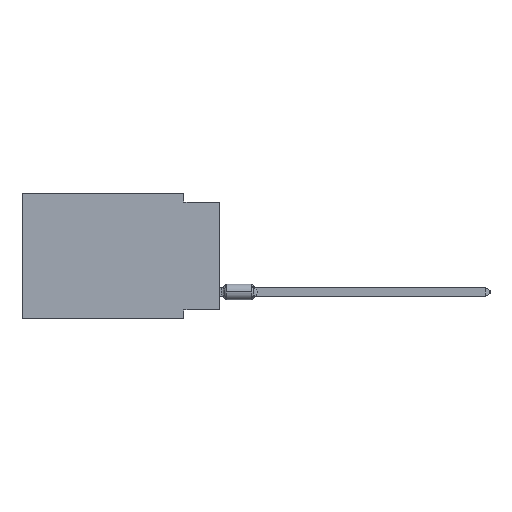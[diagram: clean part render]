
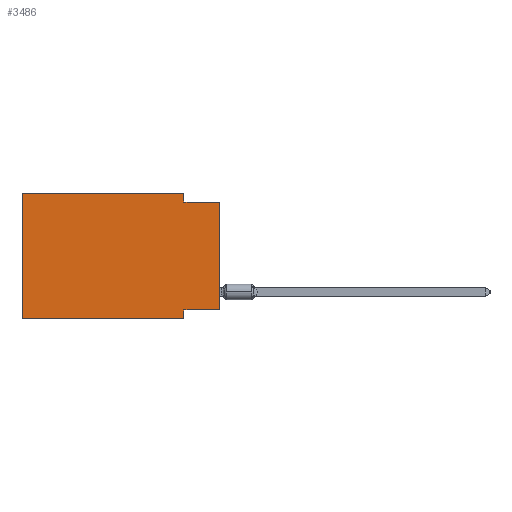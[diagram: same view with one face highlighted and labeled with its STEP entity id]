
A CAD part, left-side view. The second image highlights one B-rep face of the part: STEP entity #3486.
In plain terms, the highlighted planar face has unit normal (-1, 0, 0).
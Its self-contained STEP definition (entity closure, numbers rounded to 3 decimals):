
#558 = EDGE_CURVE ( 'NONE', #11750, #9548, #14849, .T. ) ;
#1206 = PLANE ( 'NONE',  #18500 ) ;
#1354 = DIRECTION ( 'NONE',  ( 0., -1., 0. ) ) ;
#1635 = VECTOR ( 'NONE', #8632, 1000. ) ;
#1766 = CARTESIAN_POINT ( 'NONE',  ( 0., 13.97, 0. ) ) ;
#2144 = CARTESIAN_POINT ( 'NONE',  ( 0., 2.54, -8.89 ) ) ;
#2290 = VECTOR ( 'NONE', #11818, 1000. ) ;
#2728 = CARTESIAN_POINT ( 'NONE',  ( 0., 2.54, -8.89 ) ) ;
#3170 = ORIENTED_EDGE ( 'NONE', *, *, #18254, .F. ) ;
#3486 = ADVANCED_FACE ( 'NONE', ( #5914 ), #1206, .F. ) ;
#3530 = EDGE_CURVE ( 'NONE', #15870, #7980, #17736, .T. ) ;
#3556 = LINE ( 'NONE', #18322, #11150 ) ;
#4322 = ORIENTED_EDGE ( 'NONE', *, *, #18284, .F. ) ;
#4835 = EDGE_CURVE ( 'NONE', #9548, #13205, #13509, .T. ) ;
#5208 = LINE ( 'NONE', #8612, #12692 ) ;
#5242 = CARTESIAN_POINT ( 'NONE',  ( 0., 2.54, -8.255 ) ) ;
#5760 = CARTESIAN_POINT ( 'NONE',  ( 0., 0., -0.635 ) ) ;
#5914 = FACE_OUTER_BOUND ( 'NONE', #9506, .T. ) ;
#6008 = CARTESIAN_POINT ( 'NONE',  ( 0., 2.54, 0. ) ) ;
#6281 = VECTOR ( 'NONE', #16635, 1000. ) ;
#6941 = VERTEX_POINT ( 'NONE', #5242 ) ;
#7406 = LINE ( 'NONE', #8763, #11508 ) ;
#7618 = CARTESIAN_POINT ( 'NONE',  ( 0., 0., -0.635 ) ) ;
#7980 = VERTEX_POINT ( 'NONE', #7618 ) ;
#8101 = DIRECTION ( 'NONE',  ( 0., 0., -1. ) ) ;
#8123 = ORIENTED_EDGE ( 'NONE', *, *, #8288, .T. ) ;
#8288 = EDGE_CURVE ( 'NONE', #11750, #16385, #7406, .T. ) ;
#8612 = CARTESIAN_POINT ( 'NONE',  ( 0., 0., -8.255 ) ) ;
#8632 = DIRECTION ( 'NONE',  ( 0., 0., 1. ) ) ;
#8695 = ORIENTED_EDGE ( 'NONE', *, *, #16436, .F. ) ;
#8763 = CARTESIAN_POINT ( 'NONE',  ( 0., 13.97, -8.89 ) ) ;
#8831 = DIRECTION ( 'NONE',  ( 1., 0., 0. ) ) ;
#8982 = VECTOR ( 'NONE', #1354, 1000. ) ;
#9052 = CARTESIAN_POINT ( 'NONE',  ( 0., 13.97, -8.89 ) ) ;
#9165 = VECTOR ( 'NONE', #8101, 1000. ) ;
#9413 = ORIENTED_EDGE ( 'NONE', *, *, #4835, .F. ) ;
#9506 = EDGE_LOOP ( 'NONE', ( #12546, #8695, #3170, #9413, #18606, #8123, #14599, #4322 ) ) ;
#9548 = VERTEX_POINT ( 'NONE', #14674 ) ;
#10699 = VERTEX_POINT ( 'NONE', #11994 ) ;
#11150 = VECTOR ( 'NONE', #16860, 1000. ) ;
#11508 = VECTOR ( 'NONE', #13369, 1000. ) ;
#11684 = CARTESIAN_POINT ( 'NONE',  ( 0., 0., 0. ) ) ;
#11750 = VERTEX_POINT ( 'NONE', #9052 ) ;
#11818 = DIRECTION ( 'NONE',  ( 0., 0., 1. ) ) ;
#11994 = CARTESIAN_POINT ( 'NONE',  ( 0., 2.54, -0.635 ) ) ;
#12546 = ORIENTED_EDGE ( 'NONE', *, *, #3530, .T. ) ;
#12692 = VECTOR ( 'NONE', #16058, 1000. ) ;
#12736 = EDGE_CURVE ( 'NONE', #6941, #16385, #15344, .T. ) ;
#13205 = VERTEX_POINT ( 'NONE', #6008 ) ;
#13276 = CARTESIAN_POINT ( 'NONE',  ( 0., 13.97, 0. ) ) ;
#13369 = DIRECTION ( 'NONE',  ( 0., -1., 0. ) ) ;
#13509 = LINE ( 'NONE', #1766, #6281 ) ;
#14599 = ORIENTED_EDGE ( 'NONE', *, *, #12736, .F. ) ;
#14674 = CARTESIAN_POINT ( 'NONE',  ( 0., 13.97, 0. ) ) ;
#14849 = LINE ( 'NONE', #13276, #2290 ) ;
#15344 = LINE ( 'NONE', #2144, #9165 ) ;
#15870 = VERTEX_POINT ( 'NONE', #17045 ) ;
#15931 = LINE ( 'NONE', #5760, #8982 ) ;
#16058 = DIRECTION ( 'NONE',  ( 0., 1., 0. ) ) ;
#16385 = VERTEX_POINT ( 'NONE', #2728 ) ;
#16436 = EDGE_CURVE ( 'NONE', #10699, #7980, #15931, .T. ) ;
#16472 = CARTESIAN_POINT ( 'NONE',  ( 0., 13.97, 0. ) ) ;
#16635 = DIRECTION ( 'NONE',  ( 0., -1., 0. ) ) ;
#16860 = DIRECTION ( 'NONE',  ( 0., 0., -1. ) ) ;
#17045 = CARTESIAN_POINT ( 'NONE',  ( 0., 0., -8.255 ) ) ;
#17736 = LINE ( 'NONE', #11684, #1635 ) ;
#17939 = DIRECTION ( 'NONE',  ( 0., 0., -1. ) ) ;
#18254 = EDGE_CURVE ( 'NONE', #13205, #10699, #3556, .T. ) ;
#18284 = EDGE_CURVE ( 'NONE', #15870, #6941, #5208, .T. ) ;
#18322 = CARTESIAN_POINT ( 'NONE',  ( 0., 2.54, 0. ) ) ;
#18500 = AXIS2_PLACEMENT_3D ( 'NONE', #16472, #8831, #17939 ) ;
#18606 = ORIENTED_EDGE ( 'NONE', *, *, #558, .F. ) ;
